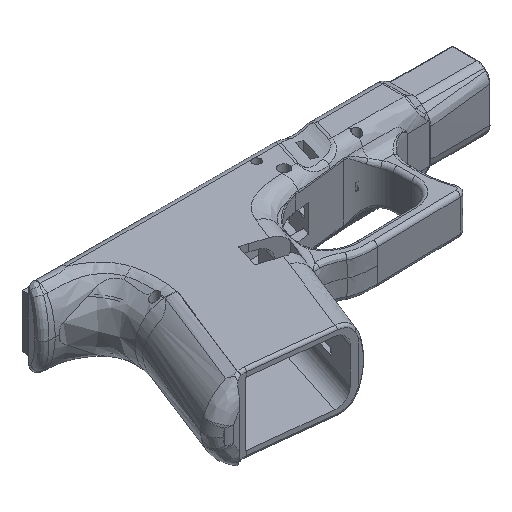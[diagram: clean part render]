
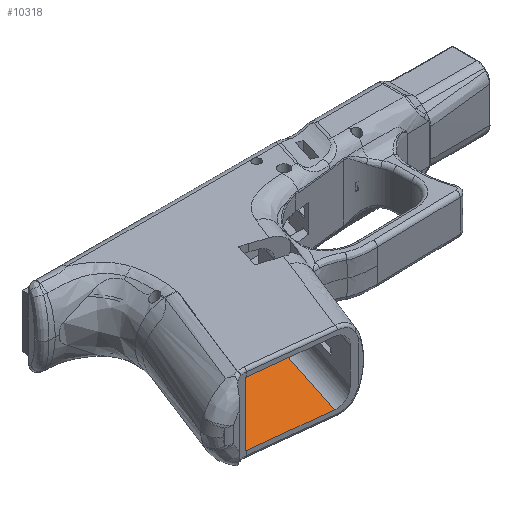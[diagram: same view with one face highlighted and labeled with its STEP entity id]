
A CAD part, isometric view. The second image highlights one B-rep face of the part: STEP entity #10318.
In plain terms, the highlighted planar face has unit normal (0, 0, 1).
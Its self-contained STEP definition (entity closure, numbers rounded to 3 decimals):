
#362=CIRCLE('',#11039,6.);
#1920=FACE_OUTER_BOUND('',#2478,.T.);
#2478=EDGE_LOOP('',(#8004,#8005,#8006,#8007,#8008,#8009,#8010,#8011,#8012,
#8013,#8014,#8015,#8016));
#2896=LINE('',#14533,#3495);
#2993=LINE('',#16967,#3592);
#3131=LINE('',#24210,#3730);
#3162=LINE('',#25904,#3761);
#3163=LINE('',#25906,#3762);
#3164=LINE('',#25908,#3763);
#3165=LINE('',#25909,#3764);
#3166=LINE('',#25911,#3765);
#3167=LINE('',#25913,#3766);
#3168=LINE('',#25914,#3767);
#3169=LINE('',#25916,#3768);
#3170=LINE('',#25917,#3769);
#3495=VECTOR('',#11792,10.);
#3592=VECTOR('',#12025,10.);
#3730=VECTOR('',#12519,10.);
#3761=VECTOR('',#12670,10.);
#3762=VECTOR('',#12671,10.);
#3763=VECTOR('',#12672,10.);
#3764=VECTOR('',#12673,10.);
#3765=VECTOR('',#12674,10.);
#3766=VECTOR('',#12675,10.);
#3767=VECTOR('',#12676,10.);
#3768=VECTOR('',#12677,10.);
#3769=VECTOR('',#12678,1000.);
#4245=VERTEX_POINT('',#14530);
#4246=VERTEX_POINT('',#14532);
#4376=VERTEX_POINT('',#16964);
#4377=VERTEX_POINT('',#16966);
#4672=VERTEX_POINT('',#24207);
#4673=VERTEX_POINT('',#24209);
#4697=VERTEX_POINT('',#24606);
#4751=VERTEX_POINT('',#25903);
#4752=VERTEX_POINT('',#25905);
#4753=VERTEX_POINT('',#25907);
#4754=VERTEX_POINT('',#25910);
#4755=VERTEX_POINT('',#25912);
#4756=VERTEX_POINT('',#25915);
#5309=EDGE_CURVE('',#4245,#4246,#2896,.F.);
#5477=EDGE_CURVE('',#4376,#4377,#2993,.F.);
#5860=EDGE_CURVE('',#4673,#4672,#3131,.T.);
#5892=EDGE_CURVE('',#4697,#4673,#362,.F.);
#5980=EDGE_CURVE('',#4751,#4246,#3162,.T.);
#5981=EDGE_CURVE('',#4752,#4245,#3163,.F.);
#5982=EDGE_CURVE('',#4753,#4752,#3164,.F.);
#5983=EDGE_CURVE('',#4377,#4753,#3165,.F.);
#5984=EDGE_CURVE('',#4754,#4376,#3166,.F.);
#5985=EDGE_CURVE('',#4755,#4754,#3167,.T.);
#5986=EDGE_CURVE('',#4697,#4755,#3168,.T.);
#5987=EDGE_CURVE('',#4756,#4672,#3169,.T.);
#5988=EDGE_CURVE('',#4756,#4751,#3170,.T.);
#8004=ORIENTED_EDGE('',*,*,#5980,.T.);
#8005=ORIENTED_EDGE('',*,*,#5309,.F.);
#8006=ORIENTED_EDGE('',*,*,#5981,.F.);
#8007=ORIENTED_EDGE('',*,*,#5982,.F.);
#8008=ORIENTED_EDGE('',*,*,#5983,.F.);
#8009=ORIENTED_EDGE('',*,*,#5477,.F.);
#8010=ORIENTED_EDGE('',*,*,#5984,.F.);
#8011=ORIENTED_EDGE('',*,*,#5985,.F.);
#8012=ORIENTED_EDGE('',*,*,#5986,.F.);
#8013=ORIENTED_EDGE('',*,*,#5892,.T.);
#8014=ORIENTED_EDGE('',*,*,#5860,.T.);
#8015=ORIENTED_EDGE('',*,*,#5987,.F.);
#8016=ORIENTED_EDGE('',*,*,#5988,.T.);
#10013=PLANE('',#11083);
#10318=ADVANCED_FACE('',(#1920),#10013,.T.);
#11039=AXIS2_PLACEMENT_3D('',#24607,#12556,#12557);
#11083=AXIS2_PLACEMENT_3D('',#25902,#12668,#12669);
#11792=DIRECTION('',(-1.,0.,0.));
#12025=DIRECTION('',(-1.,0.,0.));
#12519=DIRECTION('',(0.994,-0.111,0.));
#12556=DIRECTION('center_axis',(0.,0.,1.));
#12557=DIRECTION('ref_axis',(-0.451,0.893,0.));
#12668=DIRECTION('center_axis',(0.,0.,1.));
#12669=DIRECTION('ref_axis',(1.,0.,0.));
#12670=DIRECTION('',(0.301,0.954,0.));
#12671=DIRECTION('',(0.,-1.,0.));
#12672=DIRECTION('',(-1.,0.,0.));
#12673=DIRECTION('',(0.,1.,0.));
#12674=DIRECTION('',(-0.309,-0.951,0.));
#12675=DIRECTION('',(0.951,-0.309,0.));
#12676=DIRECTION('',(0.309,0.951,0.));
#12677=DIRECTION('',(-0.309,-0.951,0.));
#12678=DIRECTION('',(1.,0.,0.));
#14530=CARTESIAN_POINT('',(62.1,-1.5,-11.75));
#14532=CARTESIAN_POINT('',(69.764,-1.5,-11.75));
#14533=CARTESIAN_POINT('',(61.488,-1.5,-11.75));
#16964=CARTESIAN_POINT('',(47.586,-1.5,-11.75));
#16966=CARTESIAN_POINT('',(52.35,-1.5,-11.75));
#16967=CARTESIAN_POINT('',(61.488,-1.5,-11.75));
#24207=CARTESIAN_POINT('',(41.004,-72.908,-11.75));
#24209=CARTESIAN_POINT('',(11.763,-69.638,-11.75));
#24210=CARTESIAN_POINT('',(12.068,-69.672,-11.75));
#24606=CARTESIAN_POINT('',(11.46,-69.612,-11.75));
#24607=CARTESIAN_POINT('Origin',(11.096,-75.601,-11.75));
#25902=CARTESIAN_POINT('Origin',(-2.2,-1.,-11.75));
#25903=CARTESIAN_POINT('',(65.192,-16.,-11.75));
#25904=CARTESIAN_POINT('',(66.549,-11.698,-11.75));
#25905=CARTESIAN_POINT('',(62.1,-3.,-11.75));
#25906=CARTESIAN_POINT('',(62.1,-53.999,-11.75));
#25907=CARTESIAN_POINT('',(52.35,-3.,-11.75));
#25908=CARTESIAN_POINT('',(46.014,-3.,-11.75));
#25909=CARTESIAN_POINT('',(52.35,-54.999,-11.75));
#25910=CARTESIAN_POINT('',(44.828,-9.989,-11.75));
#25911=CARTESIAN_POINT('',(29.862,-56.051,-11.75));
#25912=CARTESIAN_POINT('',(32.169,-5.875,-11.75));
#25913=CARTESIAN_POINT('',(32.712,-6.052,-11.75));
#25914=CARTESIAN_POINT('',(2.312,-97.765,-11.75));
#25915=CARTESIAN_POINT('',(59.494,-16.,-11.75));
#25916=CARTESIAN_POINT('',(43.969,-63.781,-11.75));
#25917=CARTESIAN_POINT('',(0.,-16.,-11.75));
